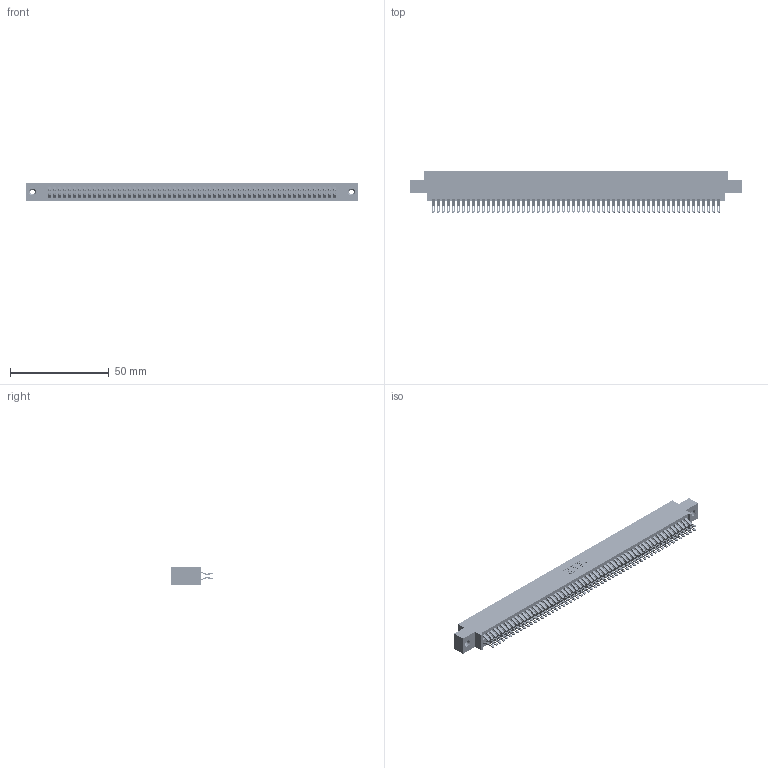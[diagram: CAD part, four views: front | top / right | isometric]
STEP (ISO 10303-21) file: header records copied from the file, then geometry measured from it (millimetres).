
FILE_DESCRIPTION (( 'STEP AP203' ), '1' );
FILE_NAME ('395-116-555-808.STEP', '2019-10-27T22:00:28', ( '' ), ( '' ), 'SwSTEP 2.0', 'SolidWorks 2016', '' );
FILE_SCHEMA (( 'CONFIG_CONTROL_DESIGN' ));
Length unit declared in the file: inch
Products named in the file (4): 395-116-555-808; 345 Part_0.170 Offset - 0.156 Dia-TI; 345-292-001_555 Tail; 345-250-001_345-250-003-102
Assembly tree (119 placements, depth 2):
  395-116-555-808
    345 Part_0.170 Offset - 0.156 Dia-TI
    345-292-001_555 Tail  x116
    345-250-001_345-250-003-102  x2
Bounding box: 168.53 x 21.13 x 9.4 mm (x, y, z)
Volume: 16736.2 mm3; surface area: 26375.9 mm2
Topology: 119 solids, 119 shells, 6686 faces, 21021 edges, 14006 vertices
Faces by surface type: plane 3712, cylinder 2958, cone 12, torus 4
Entity records: 44998 total; most frequent: CARTESIAN_POINT 7545, ORIENTED_EDGE 7442, DIRECTION 6627, EDGE_CURVE 3721, VECTOR 3317, LINE 3317, VERTEX_POINT 2476, AXIS2_PLACEMENT_3D 1655
